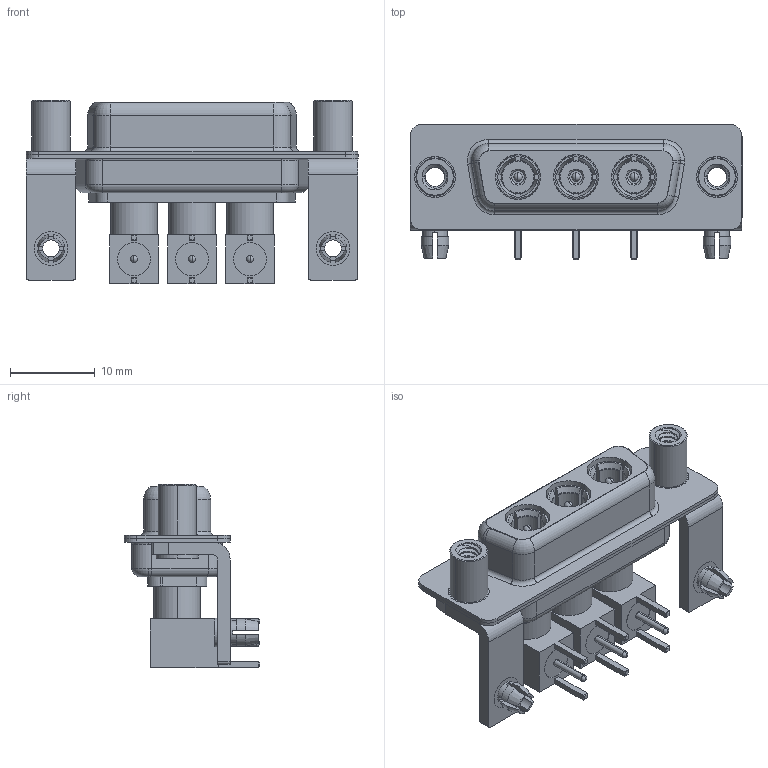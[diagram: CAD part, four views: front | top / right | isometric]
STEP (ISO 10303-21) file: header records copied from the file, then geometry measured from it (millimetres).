
FILE_DESCRIPTION (( 'STEP AP203' ), '1' );
FILE_NAME ('630-3W3-640-5T5.STEP', '2022-05-30T13:53:03', ( '' ), ( '' ), 'SwSTEP 2.0', 'SolidWorks 2020', '' );
FILE_SCHEMA (( 'CONFIG_CONTROL_DESIGN' ));
Length unit declared in the file: millimetre
Products named in the file (16): 630Combo Threaded Standoff_5; Co-Ax Plug_RA PC Tail; 630Combo Housing_3W3; Co-Ax Plug Assy_RA; 630Combo Board Lock; Insulator Pin_Straight PC Tail; 630Combo Shell Rear_15 Contacts; Insulator RA Pin; 630-3W3-640-5T5; 630Combo Stabilizer Bracket; Locking Collar; RA Back Shell; 630Combo Shell Front_15 Contacts; Pin_RA
Assembly tree (30 placements, depth 3):
  630-3W3-640-5T5
    630Combo Housing_3W3
    630Combo Shell Front_15 Contacts
    630Combo Shell Rear_15 Contacts
    630Combo Stabilizer Bracket  x2
    630Combo Board Lock  x2
    630Combo Threaded Standoff_5  x2
    Co-Ax Plug Assy_RA
      Co-Ax Plug_RA PC Tail
      Insulator Pin_Straight PC Tail
      Pin_RA
      Locking Collar
      RA Back Shell
      Insulator RA Pin
    Co-Ax Plug Assy_RA
      Co-Ax Plug_RA PC Tail
      Insulator Pin_Straight PC Tail
      Pin_RA
      Locking Collar
      RA Back Shell
      Insulator RA Pin
    Co-Ax Plug Assy_RA
      Co-Ax Plug_RA PC Tail
      Insulator Pin_Straight PC Tail
      Pin_RA
      Locking Collar
      RA Back Shell
      Insulator RA Pin
Bounding box: 39.2 x 16 x 21.61 mm (x, y, z)
Volume: 3572.4 mm3; surface area: 8914.4 mm2
Topology: 27 solids, 27 shells, 963 faces, 2372 edges, 1498 vertices
Faces by surface type: cylinder 424, plane 338, cone 105, torus 75, sphere 12, bspline 9
Entity records: 19466 total; most frequent: CARTESIAN_POINT 4957, DIRECTION 2763, ORIENTED_EDGE 2518, EDGE_CURVE 1259, AXIS2_PLACEMENT_3D 1101, VERTEX_POINT 799, EDGE_LOOP 578, VECTOR 561
